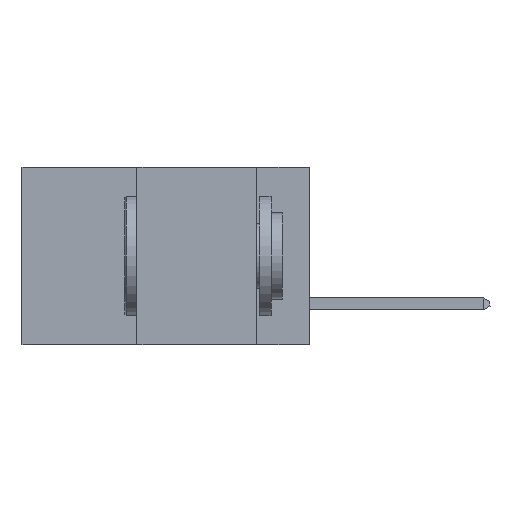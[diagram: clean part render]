
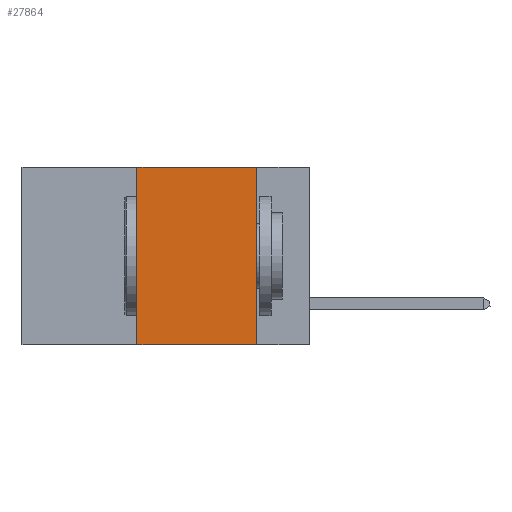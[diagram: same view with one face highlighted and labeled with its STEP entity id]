
A CAD part, left-side view. The second image highlights one B-rep face of the part: STEP entity #27864.
In plain terms, the highlighted planar face has unit normal (-1, 0, 0).
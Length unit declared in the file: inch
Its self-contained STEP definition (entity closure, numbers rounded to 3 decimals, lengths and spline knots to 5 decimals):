
#2321 = PLANE ( 'NONE',  #9273 ) ;
#2814 = CARTESIAN_POINT ( 'NONE',  ( 0., 0.11, 0. ) ) ;
#3706 = DIRECTION ( 'NONE',  ( 0., -1., 0. ) ) ;
#3813 = CARTESIAN_POINT ( 'NONE',  ( 0., 0.6, 0. ) ) ;
#4746 = VERTEX_POINT ( 'NONE', #23682 ) ;
#4825 = CARTESIAN_POINT ( 'NONE',  ( 0., 0.6, 0. ) ) ;
#5334 = DIRECTION ( 'NONE',  ( 0., 0., -1. ) ) ;
#5421 = ORIENTED_EDGE ( 'NONE', *, *, #18063, .F. ) ;
#9273 = AXIS2_PLACEMENT_3D ( 'NONE', #4825, #17113, #24392 ) ;
#9390 = LINE ( 'NONE', #12499, #22297 ) ;
#11585 = EDGE_CURVE ( 'NONE', #13218, #25964, #24562, .T. ) ;
#12499 = CARTESIAN_POINT ( 'NONE',  ( 0., 0.6, -0.37 ) ) ;
#13218 = VERTEX_POINT ( 'NONE', #16969 ) ;
#15501 = EDGE_LOOP ( 'NONE', ( #17712, #24148, #5421, #25665 ) ) ;
#15558 = CARTESIAN_POINT ( 'NONE',  ( 0., 0.36, 0. ) ) ;
#15656 = FACE_OUTER_BOUND ( 'NONE', #15501, .T. ) ;
#16969 = CARTESIAN_POINT ( 'NONE',  ( 0., 0.11, 0. ) ) ;
#17113 = DIRECTION ( 'NONE',  ( 1., 0., 0. ) ) ;
#17712 = ORIENTED_EDGE ( 'NONE', *, *, #11585, .F. ) ;
#18063 = EDGE_CURVE ( 'NONE', #23199, #4746, #22688, .T. ) ;
#18267 = CARTESIAN_POINT ( 'NONE',  ( 0., 0.36, -0.37 ) ) ;
#21951 = VECTOR ( 'NONE', #22738, 39.37008 ) ;
#22110 = DIRECTION ( 'NONE',  ( 0., -1., 0. ) ) ;
#22297 = VECTOR ( 'NONE', #22110, 39.37008 ) ;
#22342 = LINE ( 'NONE', #3813, #27296 ) ;
#22688 = LINE ( 'NONE', #15558, #21951 ) ;
#22738 = DIRECTION ( 'NONE',  ( 0., 0., 1. ) ) ;
#22923 = EDGE_CURVE ( 'NONE', #23199, #25964, #9390, .T. ) ;
#23199 = VERTEX_POINT ( 'NONE', #18267 ) ;
#23682 = CARTESIAN_POINT ( 'NONE',  ( 0., 0.36, 0. ) ) ;
#24148 = ORIENTED_EDGE ( 'NONE', *, *, #30415, .F. ) ;
#24392 = DIRECTION ( 'NONE',  ( 0., 0., -1. ) ) ;
#24562 = LINE ( 'NONE', #2814, #30265 ) ;
#25665 = ORIENTED_EDGE ( 'NONE', *, *, #22923, .T. ) ;
#25964 = VERTEX_POINT ( 'NONE', #26651 ) ;
#26651 = CARTESIAN_POINT ( 'NONE',  ( 0., 0.11, -0.37 ) ) ;
#27296 = VECTOR ( 'NONE', #3706, 39.37008 ) ;
#27864 = ADVANCED_FACE ( 'NONE', ( #15656 ), #2321, .F. ) ;
#30265 = VECTOR ( 'NONE', #5334, 39.37008 ) ;
#30415 = EDGE_CURVE ( 'NONE', #4746, #13218, #22342, .T. ) ;
